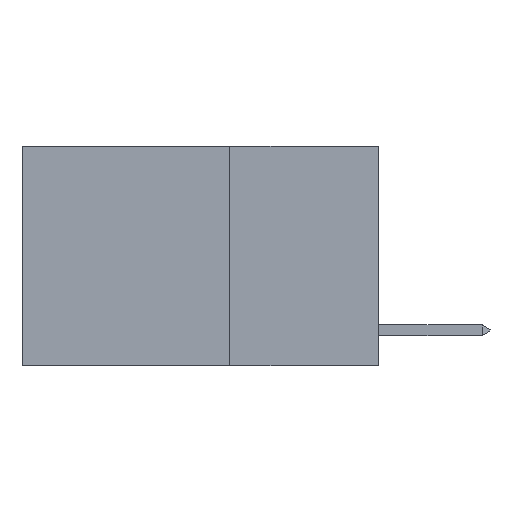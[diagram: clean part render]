
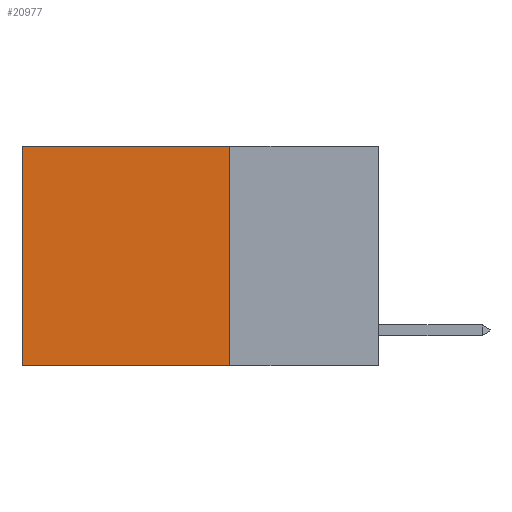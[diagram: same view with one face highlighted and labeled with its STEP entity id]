
A CAD part, left-side view. The second image highlights one B-rep face of the part: STEP entity #20977.
In plain terms, the highlighted planar face has unit normal (-1, 0, 0).
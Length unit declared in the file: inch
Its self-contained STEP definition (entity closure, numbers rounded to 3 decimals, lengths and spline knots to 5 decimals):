
#109 = EDGE_CURVE ( 'NONE', #9149, #16402, #7201, .T. ) ;
#851 = DIRECTION ( 'NONE',  ( 0., 0., -1. ) ) ;
#1387 = VERTEX_POINT ( 'NONE', #5337 ) ;
#2769 = PLANE ( 'NONE',  #10366 ) ;
#3078 = VECTOR ( 'NONE', #9941, 39.37008 ) ;
#3640 = CARTESIAN_POINT ( 'NONE',  ( 0.2625, 0.25, -0.37 ) ) ;
#5054 = CARTESIAN_POINT ( 'NONE',  ( 0.2625, 0.25, -0.37 ) ) ;
#5337 = CARTESIAN_POINT ( 'NONE',  ( 0.2625, 0.25, 0. ) ) ;
#5995 = LINE ( 'NONE', #6142, #6835 ) ;
#6068 = EDGE_CURVE ( 'NONE', #18589, #16402, #16622, .T. ) ;
#6142 = CARTESIAN_POINT ( 'NONE',  ( 0.2625, 0.25, 0. ) ) ;
#6162 = CARTESIAN_POINT ( 'NONE',  ( 0.2625, 0.25, 0. ) ) ;
#6835 = VECTOR ( 'NONE', #18460, 39.37008 ) ;
#7007 = ORIENTED_EDGE ( 'NONE', *, *, #6068, .F. ) ;
#7201 = LINE ( 'NONE', #12605, #10736 ) ;
#7540 = DIRECTION ( 'NONE',  ( 0., 0., -1. ) ) ;
#7692 = FACE_OUTER_BOUND ( 'NONE', #13817, .T. ) ;
#8763 = CARTESIAN_POINT ( 'NONE',  ( 0.2625, 0.6, 0. ) ) ;
#9149 = VERTEX_POINT ( 'NONE', #8763 ) ;
#9187 = DIRECTION ( 'NONE',  ( 0., 1., 0. ) ) ;
#9494 = DIRECTION ( 'NONE',  ( 1., 0., 0. ) ) ;
#9941 = DIRECTION ( 'NONE',  ( 0., 1., 0. ) ) ;
#10366 = AXIS2_PLACEMENT_3D ( 'NONE', #15085, #9494, #851 ) ;
#10736 = VECTOR ( 'NONE', #7540, 39.37008 ) ;
#11343 = EDGE_CURVE ( 'NONE', #1387, #9149, #17131, .T. ) ;
#12605 = CARTESIAN_POINT ( 'NONE',  ( 0.2625, 0.6, 0. ) ) ;
#13817 = EDGE_LOOP ( 'NONE', ( #21834, #7007, #19773, #17039 ) ) ;
#14412 = VECTOR ( 'NONE', #9187, 39.37008 ) ;
#15085 = CARTESIAN_POINT ( 'NONE',  ( 0.2625, 0.25, 0. ) ) ;
#16402 = VERTEX_POINT ( 'NONE', #22448 ) ;
#16622 = LINE ( 'NONE', #3640, #14412 ) ;
#17039 = ORIENTED_EDGE ( 'NONE', *, *, #11343, .T. ) ;
#17131 = LINE ( 'NONE', #6162, #3078 ) ;
#18460 = DIRECTION ( 'NONE',  ( 0., 0., -1. ) ) ;
#18589 = VERTEX_POINT ( 'NONE', #5054 ) ;
#19773 = ORIENTED_EDGE ( 'NONE', *, *, #21664, .F. ) ;
#20977 = ADVANCED_FACE ( 'NONE', ( #7692 ), #2769, .F. ) ;
#21664 = EDGE_CURVE ( 'NONE', #1387, #18589, #5995, .T. ) ;
#21834 = ORIENTED_EDGE ( 'NONE', *, *, #109, .T. ) ;
#22448 = CARTESIAN_POINT ( 'NONE',  ( 0.2625, 0.6, -0.37 ) ) ;
